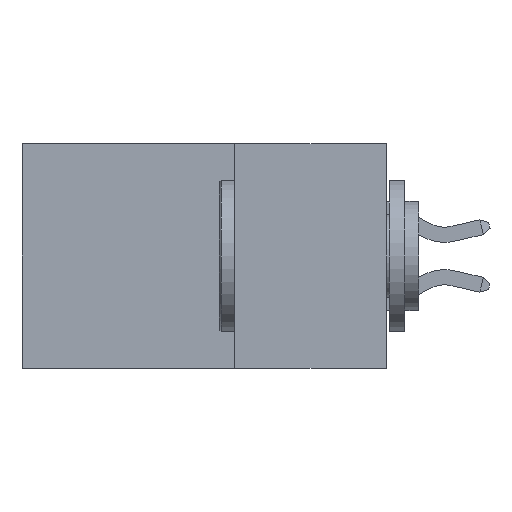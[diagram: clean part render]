
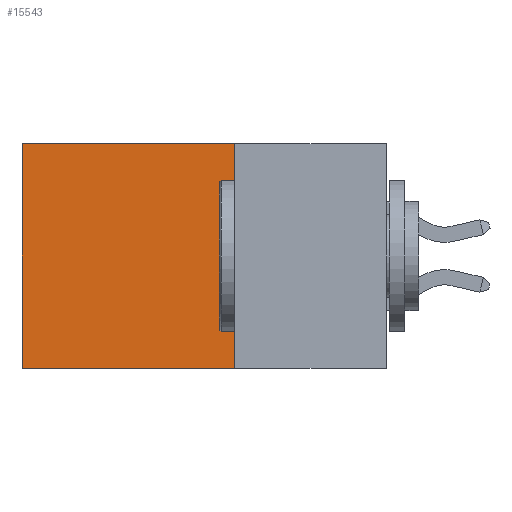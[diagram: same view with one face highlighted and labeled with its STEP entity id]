
A CAD part, left-side view. The second image highlights one B-rep face of the part: STEP entity #15543.
In plain terms, the highlighted planar face has unit normal (-1, 0, 0).
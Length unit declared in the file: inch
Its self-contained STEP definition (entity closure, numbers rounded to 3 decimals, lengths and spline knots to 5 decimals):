
#266 = PLANE ( 'NONE',  #17278 ) ;
#2884 = DIRECTION ( 'NONE',  ( 0., 0., -1. ) ) ;
#3330 = CARTESIAN_POINT ( 'NONE',  ( 0.298, 0.25, 0. ) ) ;
#3522 = VERTEX_POINT ( 'NONE', #13637 ) ;
#4634 = CARTESIAN_POINT ( 'NONE',  ( 0.298, 0.25, 0. ) ) ;
#5182 = VERTEX_POINT ( 'NONE', #30753 ) ;
#5825 = EDGE_CURVE ( 'NONE', #16948, #5182, #9781, .T. ) ;
#7935 = ORIENTED_EDGE ( 'NONE', *, *, #5825, .F. ) ;
#8239 = FACE_OUTER_BOUND ( 'NONE', #14892, .T. ) ;
#9781 = LINE ( 'NONE', #27833, #25181 ) ;
#10543 = LINE ( 'NONE', #3330, #19881 ) ;
#10696 = CARTESIAN_POINT ( 'NONE',  ( 0.298, 0.6, 0. ) ) ;
#11079 = DIRECTION ( 'NONE',  ( 0., 0., -1. ) ) ;
#11182 = LINE ( 'NONE', #13358, #22987 ) ;
#13358 = CARTESIAN_POINT ( 'NONE',  ( 0.298, 0.6, 0. ) ) ;
#13637 = CARTESIAN_POINT ( 'NONE',  ( 0.298, 0.25, 0. ) ) ;
#14892 = EDGE_LOOP ( 'NONE', ( #20016, #7935, #22047, #25696 ) ) ;
#15543 = ADVANCED_FACE ( 'NONE', ( #8239 ), #266, .F. ) ;
#16948 = VERTEX_POINT ( 'NONE', #19841 ) ;
#17278 = AXIS2_PLACEMENT_3D ( 'NONE', #20718, #18449, #2884 ) ;
#17548 = EDGE_CURVE ( 'NONE', #3522, #16948, #10543, .T. ) ;
#18449 = DIRECTION ( 'NONE',  ( 1., 0., 0. ) ) ;
#19841 = CARTESIAN_POINT ( 'NONE',  ( 0.298, 0.25, -0.37 ) ) ;
#19881 = VECTOR ( 'NONE', #11079, 39.37008 ) ;
#20016 = ORIENTED_EDGE ( 'NONE', *, *, #30973, .T. ) ;
#20718 = CARTESIAN_POINT ( 'NONE',  ( 0.298, 0.25, 0. ) ) ;
#20993 = DIRECTION ( 'NONE',  ( 0., 0., -1. ) ) ;
#21436 = LINE ( 'NONE', #4634, #33165 ) ;
#22047 = ORIENTED_EDGE ( 'NONE', *, *, #17548, .F. ) ;
#22987 = VECTOR ( 'NONE', #20993, 39.37008 ) ;
#24934 = EDGE_CURVE ( 'NONE', #3522, #28356, #21436, .T. ) ;
#25181 = VECTOR ( 'NONE', #32469, 39.37008 ) ;
#25696 = ORIENTED_EDGE ( 'NONE', *, *, #24934, .T. ) ;
#27833 = CARTESIAN_POINT ( 'NONE',  ( 0.298, 0.25, -0.37 ) ) ;
#28356 = VERTEX_POINT ( 'NONE', #10696 ) ;
#30753 = CARTESIAN_POINT ( 'NONE',  ( 0.298, 0.6, -0.37 ) ) ;
#30973 = EDGE_CURVE ( 'NONE', #28356, #5182, #11182, .T. ) ;
#32469 = DIRECTION ( 'NONE',  ( 0., 1., 0. ) ) ;
#33165 = VECTOR ( 'NONE', #33290, 39.37008 ) ;
#33290 = DIRECTION ( 'NONE',  ( 0., 1., 0. ) ) ;
